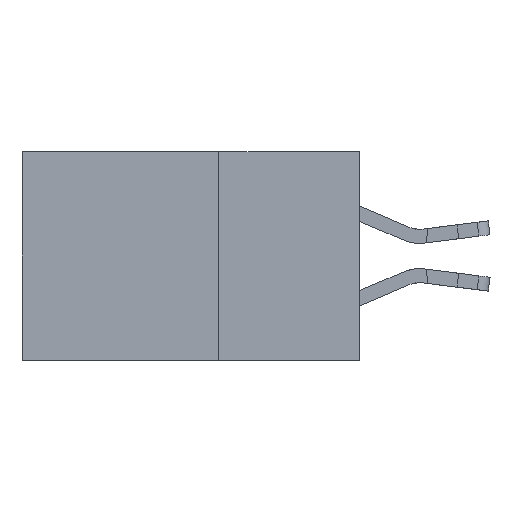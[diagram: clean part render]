
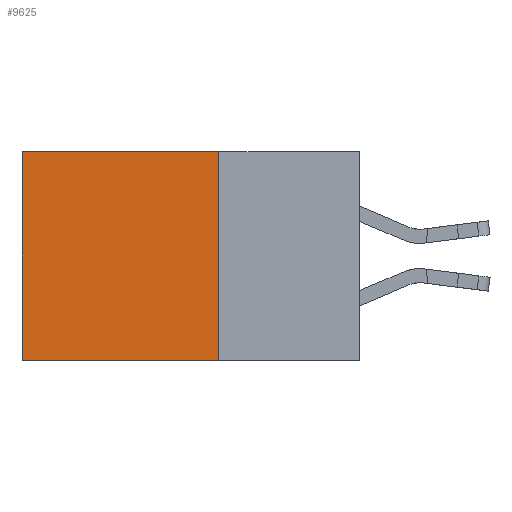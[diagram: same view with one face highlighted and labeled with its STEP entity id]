
A CAD part, left-side view. The second image highlights one B-rep face of the part: STEP entity #9625.
In plain terms, the highlighted planar face has unit normal (-1, 0, 0).
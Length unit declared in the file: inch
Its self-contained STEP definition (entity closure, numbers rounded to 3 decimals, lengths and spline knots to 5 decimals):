
#134 = CARTESIAN_POINT ( 'NONE',  ( 0.2875, 0.25, 0. ) ) ;
#817 = DIRECTION ( 'NONE',  ( 0., 0., -1. ) ) ;
#870 = DIRECTION ( 'NONE',  ( 1., 0., 0. ) ) ;
#1766 = ORIENTED_EDGE ( 'NONE', *, *, #3226, .T. ) ;
#2134 = VERTEX_POINT ( 'NONE', #134 ) ;
#2987 = DIRECTION ( 'NONE',  ( 0., 1., 0. ) ) ;
#3068 = CARTESIAN_POINT ( 'NONE',  ( 0.2875, 0.6, -0.37 ) ) ;
#3114 = EDGE_CURVE ( 'NONE', #18397, #14957, #3282, .T. ) ;
#3226 = EDGE_CURVE ( 'NONE', #2134, #18397, #5784, .T. ) ;
#3282 = LINE ( 'NONE', #22486, #21915 ) ;
#4017 = EDGE_LOOP ( 'NONE', ( #18909, #13245, #13473, #1766 ) ) ;
#4490 = LINE ( 'NONE', #13884, #12968 ) ;
#5784 = LINE ( 'NONE', #8353, #14303 ) ;
#6607 = CARTESIAN_POINT ( 'NONE',  ( 0.2875, 0.6, 0. ) ) ;
#8353 = CARTESIAN_POINT ( 'NONE',  ( 0.2875, 0.25, 0. ) ) ;
#8546 = FACE_OUTER_BOUND ( 'NONE', #4017, .T. ) ;
#9625 = ADVANCED_FACE ( 'NONE', ( #8546 ), #22543, .F. ) ;
#9774 = EDGE_CURVE ( 'NONE', #2134, #10177, #14209, .T. ) ;
#10177 = VERTEX_POINT ( 'NONE', #15014 ) ;
#10402 = DIRECTION ( 'NONE',  ( 0., 0., -1. ) ) ;
#11716 = CARTESIAN_POINT ( 'NONE',  ( 0.2875, 0.25, 0. ) ) ;
#12281 = EDGE_CURVE ( 'NONE', #10177, #14957, #4490, .T. ) ;
#12968 = VECTOR ( 'NONE', #19312, 39.37008 ) ;
#13245 = ORIENTED_EDGE ( 'NONE', *, *, #12281, .F. ) ;
#13473 = ORIENTED_EDGE ( 'NONE', *, *, #9774, .F. ) ;
#13549 = DIRECTION ( 'NONE',  ( 0., 0., -1. ) ) ;
#13884 = CARTESIAN_POINT ( 'NONE',  ( 0.2875, 0.25, -0.37 ) ) ;
#13942 = CARTESIAN_POINT ( 'NONE',  ( 0.2875, 0.25, 0. ) ) ;
#14209 = LINE ( 'NONE', #13942, #18414 ) ;
#14303 = VECTOR ( 'NONE', #2987, 39.37008 ) ;
#14957 = VERTEX_POINT ( 'NONE', #3068 ) ;
#15014 = CARTESIAN_POINT ( 'NONE',  ( 0.2875, 0.25, -0.37 ) ) ;
#18397 = VERTEX_POINT ( 'NONE', #6607 ) ;
#18414 = VECTOR ( 'NONE', #10402, 39.37008 ) ;
#18909 = ORIENTED_EDGE ( 'NONE', *, *, #3114, .T. ) ;
#19312 = DIRECTION ( 'NONE',  ( 0., 1., 0. ) ) ;
#19963 = AXIS2_PLACEMENT_3D ( 'NONE', #11716, #870, #13549 ) ;
#21915 = VECTOR ( 'NONE', #817, 39.37008 ) ;
#22486 = CARTESIAN_POINT ( 'NONE',  ( 0.2875, 0.6, 0. ) ) ;
#22543 = PLANE ( 'NONE',  #19963 ) ;
